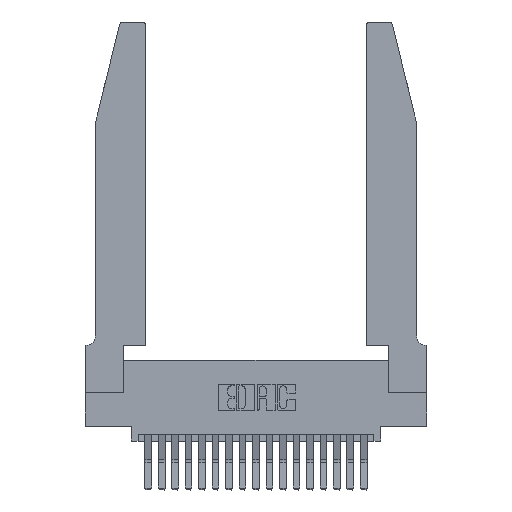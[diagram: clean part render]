
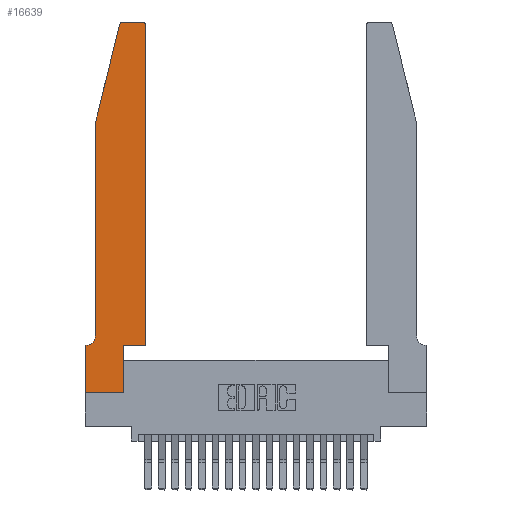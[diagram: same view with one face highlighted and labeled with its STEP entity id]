
A CAD part, top view. The second image highlights one B-rep face of the part: STEP entity #16639.
In plain terms, the highlighted planar face has unit normal (0, 0, 1).
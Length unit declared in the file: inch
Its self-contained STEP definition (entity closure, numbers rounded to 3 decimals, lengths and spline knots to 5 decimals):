
#50 = VERTEX_POINT ( 'NONE', #20577 ) ;
#390 = EDGE_CURVE ( 'NONE', #1861, #19920, #561, .T. ) ;
#421 = EDGE_CURVE ( 'NONE', #2868, #16345, #13655, .T. ) ;
#464 = LINE ( 'NONE', #15555, #18024 ) ;
#561 = LINE ( 'NONE', #11672, #10283 ) ;
#656 = ORIENTED_EDGE ( 'NONE', *, *, #4840, .T. ) ;
#787 = DIRECTION ( 'NONE',  ( 0., 0., 1. ) ) ;
#1024 = ORIENTED_EDGE ( 'NONE', *, *, #1585, .T. ) ;
#1280 = LINE ( 'NONE', #13780, #2330 ) ;
#1324 = AXIS2_PLACEMENT_3D ( 'NONE', #21024, #7875, #19572 ) ;
#1336 = ORIENTED_EDGE ( 'NONE', *, *, #2933, .T. ) ;
#1355 = VERTEX_POINT ( 'NONE', #12661 ) ;
#1585 = EDGE_CURVE ( 'NONE', #14144, #11601, #464, .T. ) ;
#1821 = LINE ( 'NONE', #15174, #19128 ) ;
#1861 = VERTEX_POINT ( 'NONE', #20995 ) ;
#1899 = CIRCLE ( 'NONE', #7772, 0.03 ) ;
#2029 = ORIENTED_EDGE ( 'NONE', *, *, #17159, .T. ) ;
#2330 = VECTOR ( 'NONE', #8760, 39.37008 ) ;
#2464 = AXIS2_PLACEMENT_3D ( 'NONE', #19182, #787, #14185 ) ;
#2470 = ORIENTED_EDGE ( 'NONE', *, *, #10328, .T. ) ;
#2481 = CARTESIAN_POINT ( 'NONE',  ( 0.0055, 0.35, 0.37 ) ) ;
#2705 = EDGE_CURVE ( 'NONE', #11278, #2868, #9079, .T. ) ;
#2735 = CARTESIAN_POINT ( 'NONE',  ( 0., 0., 0.37 ) ) ;
#2868 = VERTEX_POINT ( 'NONE', #8209 ) ;
#2933 = EDGE_CURVE ( 'NONE', #6561, #11278, #20602, .T. ) ;
#3137 = VECTOR ( 'NONE', #18334, 39.37008 ) ;
#3348 = FACE_OUTER_BOUND ( 'NONE', #18550, .T. ) ;
#3945 = PLANE ( 'NONE',  #2464 ) ;
#4041 = CARTESIAN_POINT ( 'NONE',  ( 0., 0., 0.37 ) ) ;
#4384 = DIRECTION ( 'NONE',  ( 1., 0., 0. ) ) ;
#4840 = EDGE_CURVE ( 'NONE', #16345, #50, #8490, .T. ) ;
#5033 = ORIENTED_EDGE ( 'NONE', *, *, #2705, .T. ) ;
#5914 = CARTESIAN_POINT ( 'NONE',  ( 0.4505, 0.35, 0.37 ) ) ;
#6561 = VERTEX_POINT ( 'NONE', #19138 ) ;
#7026 = DIRECTION ( 'NONE',  ( 0., 1., 0. ) ) ;
#7240 = DIRECTION ( 'NONE',  ( 1., 0., 0. ) ) ;
#7772 = AXIS2_PLACEMENT_3D ( 'NONE', #17293, #15673, #7240 ) ;
#7875 = DIRECTION ( 'NONE',  ( 0., 0., 1. ) ) ;
#7896 = ORIENTED_EDGE ( 'NONE', *, *, #10908, .T. ) ;
#8209 = CARTESIAN_POINT ( 'NONE',  ( 0., 0.35, 0.37 ) ) ;
#8490 = LINE ( 'NONE', #2735, #17911 ) ;
#8494 = ORIENTED_EDGE ( 'NONE', *, *, #421, .T. ) ;
#8760 = DIRECTION ( 'NONE',  ( 0., 1., 0. ) ) ;
#8768 = CARTESIAN_POINT ( 'NONE',  ( 0.0055, 0.42, 0.37 ) ) ;
#9079 = LINE ( 'NONE', #16079, #11697 ) ;
#9250 = VECTOR ( 'NONE', #18332, 39.37008 ) ;
#10183 = CIRCLE ( 'NONE', #1324, 0.03 ) ;
#10235 = DIRECTION ( 'NONE',  ( -1., 0., 0. ) ) ;
#10283 = VECTOR ( 'NONE', #16780, 39.37008 ) ;
#10328 = EDGE_CURVE ( 'NONE', #19226, #1355, #1821, .T. ) ;
#10693 = CARTESIAN_POINT ( 'NONE',  ( 0.0755, 2., 0.37 ) ) ;
#10746 = EDGE_CURVE ( 'NONE', #11601, #6561, #13327, .T. ) ;
#10908 = EDGE_CURVE ( 'NONE', #50, #20147, #1280, .T. ) ;
#10972 = CARTESIAN_POINT ( 'NONE',  ( 0.25487, 2.72718, 0.37 ) ) ;
#11278 = VERTEX_POINT ( 'NONE', #2481 ) ;
#11496 = ORIENTED_EDGE ( 'NONE', *, *, #10746, .T. ) ;
#11568 = CARTESIAN_POINT ( 'NONE',  ( 0.4505, 0.35, 0.37 ) ) ;
#11601 = VERTEX_POINT ( 'NONE', #17534 ) ;
#11602 = CARTESIAN_POINT ( 'NONE',  ( 0., 0., 0.37 ) ) ;
#11672 = CARTESIAN_POINT ( 'NONE',  ( 0.2605, 2.75, 0.37 ) ) ;
#11697 = VECTOR ( 'NONE', #13010, 39.37008 ) ;
#12661 = CARTESIAN_POINT ( 'NONE',  ( 0.4505, 2.72, 0.37 ) ) ;
#13010 = DIRECTION ( 'NONE',  ( -1., 0., 0. ) ) ;
#13327 = LINE ( 'NONE', #10693, #3137 ) ;
#13655 = LINE ( 'NONE', #11602, #9250 ) ;
#13780 = CARTESIAN_POINT ( 'NONE',  ( 0.2865, 0.35, 0.37 ) ) ;
#14144 = VERTEX_POINT ( 'NONE', #10972 ) ;
#14185 = DIRECTION ( 'NONE',  ( 1., 0., 0. ) ) ;
#14633 = DIRECTION ( 'NONE',  ( 1., 0., 0. ) ) ;
#15157 = DIRECTION ( 'NONE',  ( 0., 0., -1. ) ) ;
#15174 = CARTESIAN_POINT ( 'NONE',  ( 0.4505, 0.35, 0.37 ) ) ;
#15234 = ORIENTED_EDGE ( 'NONE', *, *, #16748, .T. ) ;
#15555 = CARTESIAN_POINT ( 'NONE',  ( 0.0755, 2., 0.37 ) ) ;
#15621 = LINE ( 'NONE', #5914, #15886 ) ;
#15673 = DIRECTION ( 'NONE',  ( 0., 0., 1. ) ) ;
#15768 = ORIENTED_EDGE ( 'NONE', *, *, #21237, .T. ) ;
#15886 = VECTOR ( 'NONE', #4384, 39.37008 ) ;
#16079 = CARTESIAN_POINT ( 'NONE',  ( 0.0755, 0.35, 0.37 ) ) ;
#16345 = VERTEX_POINT ( 'NONE', #4041 ) ;
#16639 = ADVANCED_FACE ( 'NONE', ( #3348 ), #3945, .T. ) ;
#16748 = EDGE_CURVE ( 'NONE', #19920, #14144, #10183, .T. ) ;
#16780 = DIRECTION ( 'NONE',  ( -1., 0., 0. ) ) ;
#17159 = EDGE_CURVE ( 'NONE', #20147, #19226, #15621, .T. ) ;
#17293 = CARTESIAN_POINT ( 'NONE',  ( 0.4205, 2.72, 0.37 ) ) ;
#17379 = AXIS2_PLACEMENT_3D ( 'NONE', #8768, #15157, #10235 ) ;
#17534 = CARTESIAN_POINT ( 'NONE',  ( 0.0755, 2., 0.37 ) ) ;
#17911 = VECTOR ( 'NONE', #14633, 39.37008 ) ;
#18024 = VECTOR ( 'NONE', #18947, 39.37008 ) ;
#18332 = DIRECTION ( 'NONE',  ( 0., -1., 0. ) ) ;
#18334 = DIRECTION ( 'NONE',  ( 0., -1., 0. ) ) ;
#18550 = EDGE_LOOP ( 'NONE', ( #21029, #15234, #1024, #11496, #1336, #5033, #8494, #656, #7896, #2029, #2470, #15768 ) ) ;
#18947 = DIRECTION ( 'NONE',  ( -0.239, -0.971, 0. ) ) ;
#19128 = VECTOR ( 'NONE', #7026, 39.37008 ) ;
#19138 = CARTESIAN_POINT ( 'NONE',  ( 0.0755, 0.42, 0.37 ) ) ;
#19182 = CARTESIAN_POINT ( 'NONE',  ( 0., 0.35, 0.37 ) ) ;
#19226 = VERTEX_POINT ( 'NONE', #11568 ) ;
#19572 = DIRECTION ( 'NONE',  ( 1., 0., 0. ) ) ;
#19920 = VERTEX_POINT ( 'NONE', #21653 ) ;
#20147 = VERTEX_POINT ( 'NONE', #21000 ) ;
#20577 = CARTESIAN_POINT ( 'NONE',  ( 0.2865, 0., 0.37 ) ) ;
#20602 = CIRCLE ( 'NONE', #17379, 0.07 ) ;
#20995 = CARTESIAN_POINT ( 'NONE',  ( 0.4205, 2.75, 0.37 ) ) ;
#21000 = CARTESIAN_POINT ( 'NONE',  ( 0.2865, 0.35, 0.37 ) ) ;
#21024 = CARTESIAN_POINT ( 'NONE',  ( 0.284, 2.72, 0.37 ) ) ;
#21029 = ORIENTED_EDGE ( 'NONE', *, *, #390, .T. ) ;
#21237 = EDGE_CURVE ( 'NONE', #1355, #1861, #1899, .T. ) ;
#21653 = CARTESIAN_POINT ( 'NONE',  ( 0.284, 2.75, 0.37 ) ) ;
